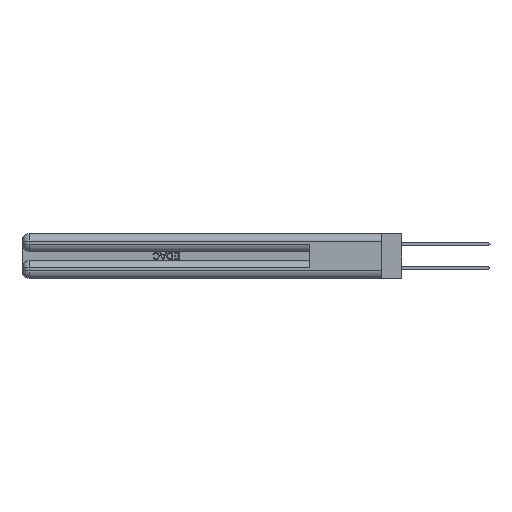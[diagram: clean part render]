
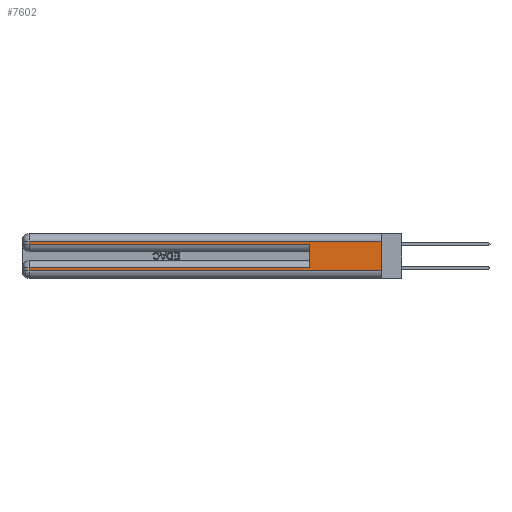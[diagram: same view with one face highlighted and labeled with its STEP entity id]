
A CAD part, left-side view. The second image highlights one B-rep face of the part: STEP entity #7602.
In plain terms, the highlighted planar face has unit normal (-1, 0, 0).
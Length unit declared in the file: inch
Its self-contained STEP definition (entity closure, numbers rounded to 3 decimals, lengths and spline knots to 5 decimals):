
#51 = VERTEX_POINT ( 'NONE', #38807 ) ;
#624 = VECTOR ( 'NONE', #4268, 39.37008 ) ;
#1255 = EDGE_CURVE ( 'NONE', #38209, #44573, #23713, .T. ) ;
#1745 = LINE ( 'NONE', #12599, #41148 ) ;
#2866 = VECTOR ( 'NONE', #32412, 39.37008 ) ;
#2897 = VERTEX_POINT ( 'NONE', #12007 ) ;
#2969 = DIRECTION ( 'NONE',  ( 0., 1., 0. ) ) ;
#3142 = CARTESIAN_POINT ( 'NONE',  ( 0., 0.6, 0.085 ) ) ;
#3342 = ORIENTED_EDGE ( 'NONE', *, *, #11381, .T. ) ;
#3345 = DIRECTION ( 'NONE',  ( 0., 0., -1. ) ) ;
#3761 = VECTOR ( 'NONE', #3934, 39.37008 ) ;
#3934 = DIRECTION ( 'NONE',  ( 0., 0., -1. ) ) ;
#4268 = DIRECTION ( 'NONE',  ( 0., 0., -1. ) ) ;
#6725 = CARTESIAN_POINT ( 'NONE',  ( 0., 0., 0.06 ) ) ;
#7602 = ADVANCED_FACE ( 'NONE', ( #37762 ), #7960, .F. ) ;
#7809 = DIRECTION ( 'NONE',  ( 0., 0., -1. ) ) ;
#7960 = PLANE ( 'NONE',  #45215 ) ;
#9882 = DIRECTION ( 'NONE',  ( 0., 1., 0. ) ) ;
#10016 = CARTESIAN_POINT ( 'NONE',  ( 0., 0., 0.37 ) ) ;
#10107 = CARTESIAN_POINT ( 'NONE',  ( 0., 0., 0.085 ) ) ;
#10592 = VECTOR ( 'NONE', #9882, 39.37008 ) ;
#11110 = ORIENTED_EDGE ( 'NONE', *, *, #29664, .F. ) ;
#11381 = EDGE_CURVE ( 'NONE', #2897, #42706, #27210, .T. ) ;
#11486 = EDGE_CURVE ( 'NONE', #26397, #38209, #11720, .T. ) ;
#11533 = CARTESIAN_POINT ( 'NONE',  ( 0., 0., 0.37 ) ) ;
#11720 = LINE ( 'NONE', #24278, #10592 ) ;
#12007 = CARTESIAN_POINT ( 'NONE',  ( 0., 2.94, 0.085 ) ) ;
#12599 = CARTESIAN_POINT ( 'NONE',  ( 0., 0., 0.285 ) ) ;
#14367 = LINE ( 'NONE', #6725, #17715 ) ;
#15769 = CARTESIAN_POINT ( 'NONE',  ( 0., 0., 0.06 ) ) ;
#16528 = EDGE_CURVE ( 'NONE', #44573, #51, #1745, .T. ) ;
#17380 = LINE ( 'NONE', #10107, #20139 ) ;
#17715 = VECTOR ( 'NONE', #28377, 39.37008 ) ;
#17879 = LINE ( 'NONE', #32094, #2866 ) ;
#17891 = ORIENTED_EDGE ( 'NONE', *, *, #11486, .T. ) ;
#18517 = DIRECTION ( 'NONE',  ( 1., 0., 0. ) ) ;
#20139 = VECTOR ( 'NONE', #2969, 39.37008 ) ;
#20573 = VECTOR ( 'NONE', #3345, 39.37008 ) ;
#20924 = CARTESIAN_POINT ( 'NONE',  ( 0., 0., 0.31 ) ) ;
#23024 = EDGE_CURVE ( 'NONE', #26397, #34197, #27221, .T. ) ;
#23713 = LINE ( 'NONE', #25298, #3761 ) ;
#24278 = CARTESIAN_POINT ( 'NONE',  ( 0., 0., 0.31 ) ) ;
#24713 = ORIENTED_EDGE ( 'NONE', *, *, #1255, .T. ) ;
#25108 = ORIENTED_EDGE ( 'NONE', *, *, #44676, .T. ) ;
#25298 = CARTESIAN_POINT ( 'NONE',  ( 0., 2.94, 0.37 ) ) ;
#26397 = VERTEX_POINT ( 'NONE', #20924 ) ;
#26682 = DIRECTION ( 'NONE',  ( 0., -1., 0. ) ) ;
#27210 = LINE ( 'NONE', #31263, #624 ) ;
#27221 = LINE ( 'NONE', #10016, #20573 ) ;
#28377 = DIRECTION ( 'NONE',  ( 0., -1., 0. ) ) ;
#29664 = EDGE_CURVE ( 'NONE', #30285, #51, #17879, .T. ) ;
#29702 = ORIENTED_EDGE ( 'NONE', *, *, #23024, .F. ) ;
#30285 = VERTEX_POINT ( 'NONE', #3142 ) ;
#30311 = EDGE_CURVE ( 'NONE', #42706, #34197, #14367, .T. ) ;
#31263 = CARTESIAN_POINT ( 'NONE',  ( 0., 2.94, 0.37 ) ) ;
#32094 = CARTESIAN_POINT ( 'NONE',  ( 0., 0.6, 0.145 ) ) ;
#32298 = EDGE_LOOP ( 'NONE', ( #29702, #17891, #24713, #33019, #11110, #25108, #3342, #37924 ) ) ;
#32412 = DIRECTION ( 'NONE',  ( 0., 0., 1. ) ) ;
#33019 = ORIENTED_EDGE ( 'NONE', *, *, #16528, .T. ) ;
#33342 = CARTESIAN_POINT ( 'NONE',  ( 0., 2.94, 0.31 ) ) ;
#33632 = CARTESIAN_POINT ( 'NONE',  ( 0., 2.94, 0.285 ) ) ;
#34197 = VERTEX_POINT ( 'NONE', #15769 ) ;
#37762 = FACE_OUTER_BOUND ( 'NONE', #32298, .T. ) ;
#37924 = ORIENTED_EDGE ( 'NONE', *, *, #30311, .T. ) ;
#38209 = VERTEX_POINT ( 'NONE', #33342 ) ;
#38807 = CARTESIAN_POINT ( 'NONE',  ( 0., 0.6, 0.285 ) ) ;
#41148 = VECTOR ( 'NONE', #26682, 39.37008 ) ;
#42706 = VERTEX_POINT ( 'NONE', #45277 ) ;
#44573 = VERTEX_POINT ( 'NONE', #33632 ) ;
#44676 = EDGE_CURVE ( 'NONE', #30285, #2897, #17380, .T. ) ;
#45215 = AXIS2_PLACEMENT_3D ( 'NONE', #11533, #18517, #7809 ) ;
#45277 = CARTESIAN_POINT ( 'NONE',  ( 0., 2.94, 0.06 ) ) ;
